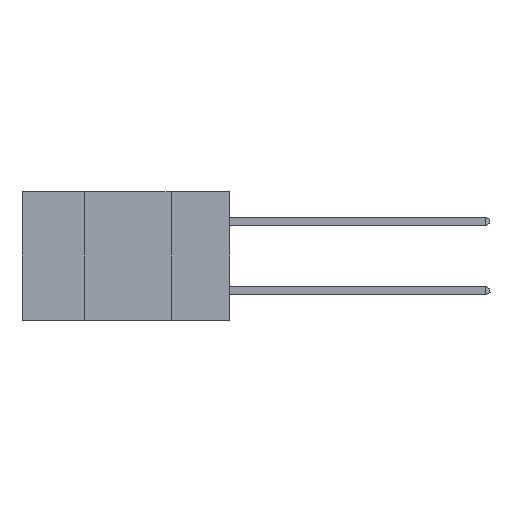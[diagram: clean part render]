
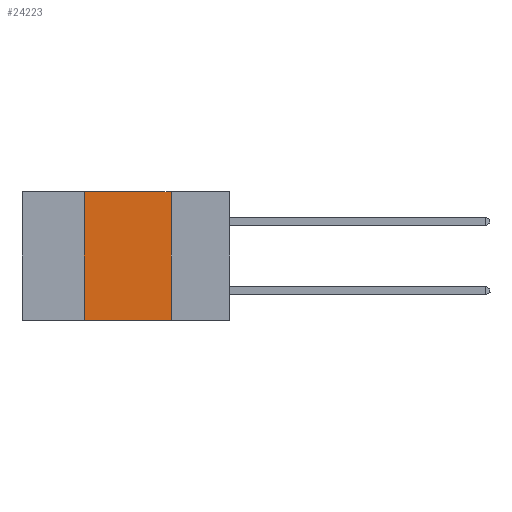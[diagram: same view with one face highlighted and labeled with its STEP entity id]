
A CAD part, left-side view. The second image highlights one B-rep face of the part: STEP entity #24223.
In plain terms, the highlighted planar face has unit normal (-1, 0, 0).
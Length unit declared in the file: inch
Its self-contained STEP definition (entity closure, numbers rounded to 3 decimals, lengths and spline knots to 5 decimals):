
#873 = CARTESIAN_POINT ( 'NONE',  ( 0., 0.42, 0. ) ) ;
#1566 = CARTESIAN_POINT ( 'NONE',  ( 0., 0.6, 0. ) ) ;
#1585 = CARTESIAN_POINT ( 'NONE',  ( 0., 0.42, -0.37 ) ) ;
#1709 = ORIENTED_EDGE ( 'NONE', *, *, #19276, .F. ) ;
#1954 = CARTESIAN_POINT ( 'NONE',  ( 0., 0.6, 0. ) ) ;
#4030 = DIRECTION ( 'NONE',  ( 0., 0., -1. ) ) ;
#4543 = CARTESIAN_POINT ( 'NONE',  ( 0., 0.17, 0. ) ) ;
#5014 = VERTEX_POINT ( 'NONE', #873 ) ;
#5887 = ORIENTED_EDGE ( 'NONE', *, *, #18520, .F. ) ;
#6219 = VECTOR ( 'NONE', #7601, 39.37008 ) ;
#6475 = FACE_OUTER_BOUND ( 'NONE', #18339, .T. ) ;
#7152 = DIRECTION ( 'NONE',  ( 0., 0., 1. ) ) ;
#7601 = DIRECTION ( 'NONE',  ( 0., 0., -1. ) ) ;
#8039 = VECTOR ( 'NONE', #9624, 39.37008 ) ;
#8673 = LINE ( 'NONE', #1566, #8039 ) ;
#9624 = DIRECTION ( 'NONE',  ( 0., -1., 0. ) ) ;
#10885 = LINE ( 'NONE', #19280, #6219 ) ;
#12368 = VECTOR ( 'NONE', #7152, 39.37008 ) ;
#12566 = DIRECTION ( 'NONE',  ( 0., -1., 0. ) ) ;
#13023 = LINE ( 'NONE', #24127, #18181 ) ;
#13632 = ORIENTED_EDGE ( 'NONE', *, *, #22371, .T. ) ;
#14976 = AXIS2_PLACEMENT_3D ( 'NONE', #1954, #15934, #4030 ) ;
#15934 = DIRECTION ( 'NONE',  ( 1., 0., 0. ) ) ;
#16949 = LINE ( 'NONE', #20752, #12368 ) ;
#17567 = ORIENTED_EDGE ( 'NONE', *, *, #19782, .F. ) ;
#17940 = VERTEX_POINT ( 'NONE', #1585 ) ;
#18181 = VECTOR ( 'NONE', #12566, 39.37008 ) ;
#18339 = EDGE_LOOP ( 'NONE', ( #5887, #1709, #17567, #13632 ) ) ;
#18520 = EDGE_CURVE ( 'NONE', #22365, #22603, #10885, .T. ) ;
#19276 = EDGE_CURVE ( 'NONE', #5014, #22365, #8673, .T. ) ;
#19280 = CARTESIAN_POINT ( 'NONE',  ( 0., 0.17, 0. ) ) ;
#19782 = EDGE_CURVE ( 'NONE', #17940, #5014, #16949, .T. ) ;
#20752 = CARTESIAN_POINT ( 'NONE',  ( 0., 0.42, 0. ) ) ;
#21595 = PLANE ( 'NONE',  #14976 ) ;
#22365 = VERTEX_POINT ( 'NONE', #4543 ) ;
#22371 = EDGE_CURVE ( 'NONE', #17940, #22603, #13023, .T. ) ;
#22603 = VERTEX_POINT ( 'NONE', #24796 ) ;
#24127 = CARTESIAN_POINT ( 'NONE',  ( 0., 0.6, -0.37 ) ) ;
#24223 = ADVANCED_FACE ( 'NONE', ( #6475 ), #21595, .F. ) ;
#24796 = CARTESIAN_POINT ( 'NONE',  ( 0., 0.17, -0.37 ) ) ;
